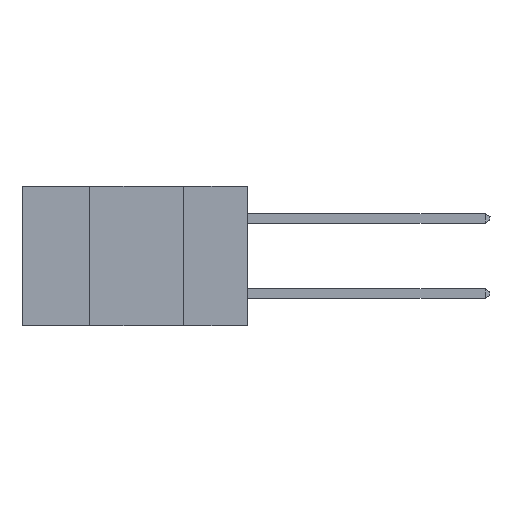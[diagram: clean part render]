
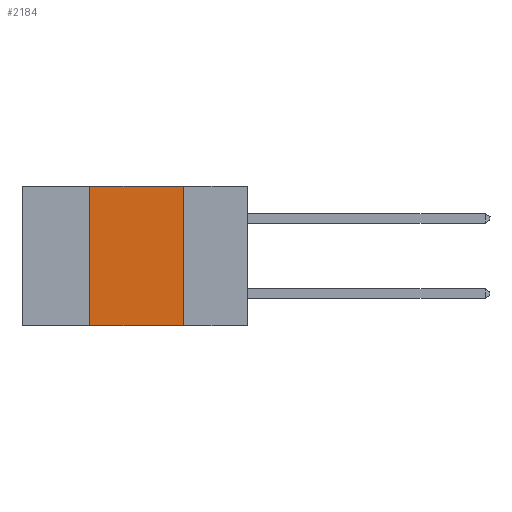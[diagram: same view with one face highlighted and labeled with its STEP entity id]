
A CAD part, left-side view. The second image highlights one B-rep face of the part: STEP entity #2184.
In plain terms, the highlighted planar face has unit normal (-1, 0, 0).
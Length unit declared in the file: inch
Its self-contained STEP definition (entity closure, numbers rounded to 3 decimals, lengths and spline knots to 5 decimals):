
#585 = CARTESIAN_POINT ( 'NONE',  ( 0., 0.17, -0.37 ) ) ;
#680 = EDGE_CURVE ( 'NONE', #17096, #15401, #11551, .T. ) ;
#1060 = VECTOR ( 'NONE', #6154, 39.37008 ) ;
#2184 = ADVANCED_FACE ( 'NONE', ( #2917 ), #10161, .F. ) ;
#2337 = DIRECTION ( 'NONE',  ( 0., 0., -1. ) ) ;
#2917 = FACE_OUTER_BOUND ( 'NONE', #22427, .T. ) ;
#3208 = VERTEX_POINT ( 'NONE', #13940 ) ;
#4321 = DIRECTION ( 'NONE',  ( 0., 0., -1. ) ) ;
#4455 = CARTESIAN_POINT ( 'NONE',  ( 0., 0.42, 0. ) ) ;
#4768 = CARTESIAN_POINT ( 'NONE',  ( 0., 0.42, -0.37 ) ) ;
#4858 = VECTOR ( 'NONE', #11756, 39.37008 ) ;
#5108 = VECTOR ( 'NONE', #2337, 39.37008 ) ;
#5511 = EDGE_CURVE ( 'NONE', #15401, #16246, #9695, .T. ) ;
#6030 = ORIENTED_EDGE ( 'NONE', *, *, #11612, .T. ) ;
#6154 = DIRECTION ( 'NONE',  ( 0., -1., 0. ) ) ;
#6312 = AXIS2_PLACEMENT_3D ( 'NONE', #6424, #17201, #4321 ) ;
#6330 = CARTESIAN_POINT ( 'NONE',  ( 0., 0.17, 0. ) ) ;
#6424 = CARTESIAN_POINT ( 'NONE',  ( 0., 0.6, 0. ) ) ;
#6575 = ORIENTED_EDGE ( 'NONE', *, *, #17781, .F. ) ;
#7595 = CARTESIAN_POINT ( 'NONE',  ( 0., 0.6, 0. ) ) ;
#8312 = ORIENTED_EDGE ( 'NONE', *, *, #680, .F. ) ;
#9695 = LINE ( 'NONE', #585, #5108 ) ;
#10103 = LINE ( 'NONE', #13387, #4858 ) ;
#10161 = PLANE ( 'NONE',  #6312 ) ;
#11551 = LINE ( 'NONE', #7595, #1060 ) ;
#11612 = EDGE_CURVE ( 'NONE', #3208, #16246, #10103, .T. ) ;
#11756 = DIRECTION ( 'NONE',  ( 0., -1., 0. ) ) ;
#11925 = DIRECTION ( 'NONE',  ( 0., 0., 1. ) ) ;
#13387 = CARTESIAN_POINT ( 'NONE',  ( 0., 0.6, -0.37 ) ) ;
#13940 = CARTESIAN_POINT ( 'NONE',  ( 0., 0.42, -0.37 ) ) ;
#15401 = VERTEX_POINT ( 'NONE', #6330 ) ;
#16246 = VERTEX_POINT ( 'NONE', #20198 ) ;
#17096 = VERTEX_POINT ( 'NONE', #4455 ) ;
#17201 = DIRECTION ( 'NONE',  ( 1., 0., 0. ) ) ;
#17781 = EDGE_CURVE ( 'NONE', #3208, #17096, #20824, .T. ) ;
#19918 = ORIENTED_EDGE ( 'NONE', *, *, #5511, .F. ) ;
#20198 = CARTESIAN_POINT ( 'NONE',  ( 0., 0.17, -0.37 ) ) ;
#20824 = LINE ( 'NONE', #4768, #22187 ) ;
#22187 = VECTOR ( 'NONE', #11925, 39.37008 ) ;
#22427 = EDGE_LOOP ( 'NONE', ( #19918, #8312, #6575, #6030 ) ) ;
